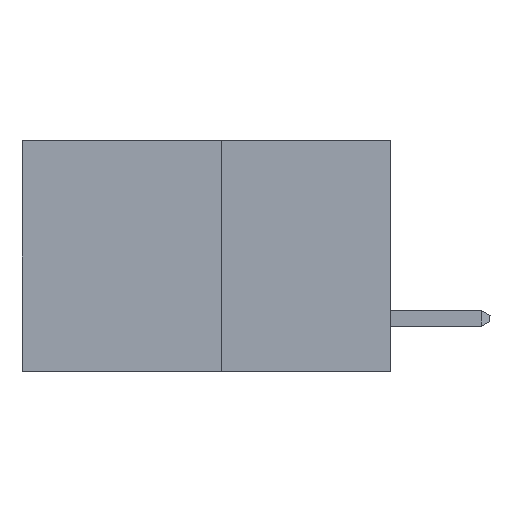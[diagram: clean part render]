
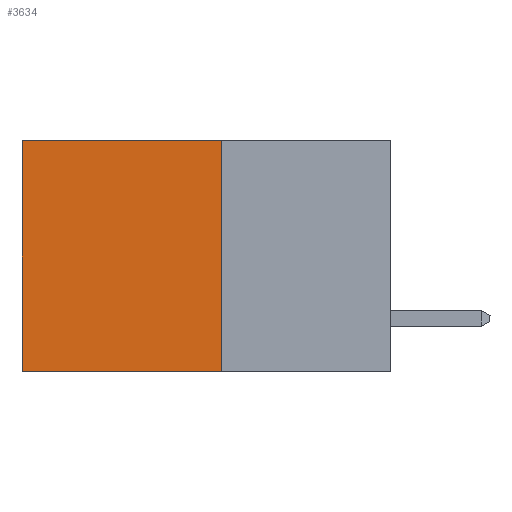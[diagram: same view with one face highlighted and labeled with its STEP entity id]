
A CAD part, left-side view. The second image highlights one B-rep face of the part: STEP entity #3634.
In plain terms, the highlighted planar face has unit normal (-1, 0, 0).
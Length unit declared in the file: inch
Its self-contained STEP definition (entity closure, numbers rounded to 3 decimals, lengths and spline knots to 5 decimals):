
#594 = ORIENTED_EDGE ( 'NONE', *, *, #15411, .F. ) ;
#1663 = CARTESIAN_POINT ( 'NONE',  ( 0.277, 0.27, 0. ) ) ;
#2910 = VERTEX_POINT ( 'NONE', #12971 ) ;
#2961 = DIRECTION ( 'NONE',  ( 0., 1., 0. ) ) ;
#3556 = CARTESIAN_POINT ( 'NONE',  ( 0.277, 0.27, -0.37 ) ) ;
#3634 = ADVANCED_FACE ( 'NONE', ( #7768 ), #10024, .F. ) ;
#4025 = DIRECTION ( 'NONE',  ( 0., 0., -1. ) ) ;
#4053 = VECTOR ( 'NONE', #4815, 39.37008 ) ;
#4096 = ORIENTED_EDGE ( 'NONE', *, *, #9403, .T. ) ;
#4338 = CARTESIAN_POINT ( 'NONE',  ( 0.277, 0.59, 0. ) ) ;
#4452 = LINE ( 'NONE', #1663, #10452 ) ;
#4795 = CARTESIAN_POINT ( 'NONE',  ( 0.277, 0.27, -0.37 ) ) ;
#4815 = DIRECTION ( 'NONE',  ( 0., 1., 0. ) ) ;
#5400 = LINE ( 'NONE', #5536, #15074 ) ;
#5536 = CARTESIAN_POINT ( 'NONE',  ( 0.277, 0.59, -0.37 ) ) ;
#6042 = DIRECTION ( 'NONE',  ( 0., 0., -1. ) ) ;
#6495 = LINE ( 'NONE', #4795, #15369 ) ;
#6607 = ORIENTED_EDGE ( 'NONE', *, *, #10906, .F. ) ;
#7360 = ORIENTED_EDGE ( 'NONE', *, *, #9953, .T. ) ;
#7376 = LINE ( 'NONE', #3556, #4053 ) ;
#7768 = FACE_OUTER_BOUND ( 'NONE', #14999, .T. ) ;
#8875 = CARTESIAN_POINT ( 'NONE',  ( 0.277, 0.27, -0.37 ) ) ;
#9036 = AXIS2_PLACEMENT_3D ( 'NONE', #8875, #11198, #4025 ) ;
#9403 = EDGE_CURVE ( 'NONE', #2910, #14045, #4452, .T. ) ;
#9564 = CARTESIAN_POINT ( 'NONE',  ( 0.277, 0.27, -0.37 ) ) ;
#9953 = EDGE_CURVE ( 'NONE', #14045, #11491, #5400, .T. ) ;
#10024 = PLANE ( 'NONE',  #9036 ) ;
#10230 = VERTEX_POINT ( 'NONE', #9564 ) ;
#10452 = VECTOR ( 'NONE', #2961, 39.37008 ) ;
#10906 = EDGE_CURVE ( 'NONE', #10230, #11491, #7376, .T. ) ;
#11198 = DIRECTION ( 'NONE',  ( 1., 0., 0. ) ) ;
#11491 = VERTEX_POINT ( 'NONE', #15180 ) ;
#12971 = CARTESIAN_POINT ( 'NONE',  ( 0.277, 0.27, 0. ) ) ;
#13701 = DIRECTION ( 'NONE',  ( 0., 0., -1. ) ) ;
#14045 = VERTEX_POINT ( 'NONE', #4338 ) ;
#14999 = EDGE_LOOP ( 'NONE', ( #7360, #6607, #594, #4096 ) ) ;
#15074 = VECTOR ( 'NONE', #13701, 39.37008 ) ;
#15180 = CARTESIAN_POINT ( 'NONE',  ( 0.277, 0.59, -0.37 ) ) ;
#15369 = VECTOR ( 'NONE', #6042, 39.37008 ) ;
#15411 = EDGE_CURVE ( 'NONE', #2910, #10230, #6495, .T. ) ;
